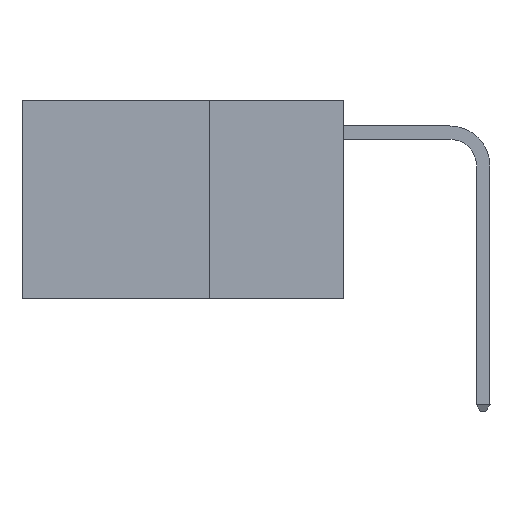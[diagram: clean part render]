
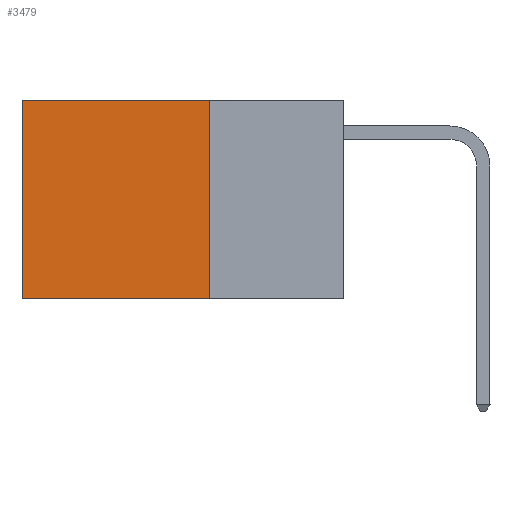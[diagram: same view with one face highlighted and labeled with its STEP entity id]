
A CAD part, left-side view. The second image highlights one B-rep face of the part: STEP entity #3479.
In plain terms, the highlighted planar face has unit normal (-1, 0, 0).
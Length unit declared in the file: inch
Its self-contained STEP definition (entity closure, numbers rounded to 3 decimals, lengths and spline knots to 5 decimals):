
#245 = CARTESIAN_POINT ( 'NONE',  ( 0.2625, 0.25, 0. ) ) ;
#851 = CARTESIAN_POINT ( 'NONE',  ( 0.2625, 0.25, 0. ) ) ;
#1081 = CARTESIAN_POINT ( 'NONE',  ( 0.2625, 0.25, -0.37 ) ) ;
#1636 = EDGE_CURVE ( 'NONE', #7985, #4533, #8687, .T. ) ;
#1965 = ORIENTED_EDGE ( 'NONE', *, *, #3971, .F. ) ;
#2007 = VECTOR ( 'NONE', #9837, 39.37008 ) ;
#2328 = VERTEX_POINT ( 'NONE', #5694 ) ;
#2361 = EDGE_LOOP ( 'NONE', ( #8353, #6186, #1965, #7417 ) ) ;
#3282 = FACE_OUTER_BOUND ( 'NONE', #2361, .T. ) ;
#3479 = ADVANCED_FACE ( 'NONE', ( #3282 ), #8121, .F. ) ;
#3773 = DIRECTION ( 'NONE',  ( 0., 0., -1. ) ) ;
#3814 = CARTESIAN_POINT ( 'NONE',  ( 0.2625, 0.25, -0.37 ) ) ;
#3971 = EDGE_CURVE ( 'NONE', #2328, #7985, #7088, .T. ) ;
#4353 = DIRECTION ( 'NONE',  ( 0., 0., -1. ) ) ;
#4533 = VERTEX_POINT ( 'NONE', #7923 ) ;
#4677 = VERTEX_POINT ( 'NONE', #10766 ) ;
#4762 = VECTOR ( 'NONE', #9611, 39.37008 ) ;
#4775 = VECTOR ( 'NONE', #7834, 39.37008 ) ;
#4884 = AXIS2_PLACEMENT_3D ( 'NONE', #245, #8974, #3773 ) ;
#5694 = CARTESIAN_POINT ( 'NONE',  ( 0.2625, 0.25, 0. ) ) ;
#6186 = ORIENTED_EDGE ( 'NONE', *, *, #1636, .F. ) ;
#6950 = CARTESIAN_POINT ( 'NONE',  ( 0.2625, 0.6, 0. ) ) ;
#7088 = LINE ( 'NONE', #851, #4762 ) ;
#7100 = LINE ( 'NONE', #11296, #4775 ) ;
#7417 = ORIENTED_EDGE ( 'NONE', *, *, #9605, .T. ) ;
#7519 = VECTOR ( 'NONE', #4353, 39.37008 ) ;
#7834 = DIRECTION ( 'NONE',  ( 0., 1., 0. ) ) ;
#7923 = CARTESIAN_POINT ( 'NONE',  ( 0.2625, 0.6, -0.37 ) ) ;
#7985 = VERTEX_POINT ( 'NONE', #3814 ) ;
#8121 = PLANE ( 'NONE',  #4884 ) ;
#8353 = ORIENTED_EDGE ( 'NONE', *, *, #10389, .T. ) ;
#8687 = LINE ( 'NONE', #1081, #2007 ) ;
#8974 = DIRECTION ( 'NONE',  ( 1., 0., 0. ) ) ;
#9605 = EDGE_CURVE ( 'NONE', #2328, #4677, #7100, .T. ) ;
#9611 = DIRECTION ( 'NONE',  ( 0., 0., -1. ) ) ;
#9830 = LINE ( 'NONE', #6950, #7519 ) ;
#9837 = DIRECTION ( 'NONE',  ( 0., 1., 0. ) ) ;
#10389 = EDGE_CURVE ( 'NONE', #4677, #4533, #9830, .T. ) ;
#10766 = CARTESIAN_POINT ( 'NONE',  ( 0.2625, 0.6, 0. ) ) ;
#11296 = CARTESIAN_POINT ( 'NONE',  ( 0.2625, 0.25, 0. ) ) ;
